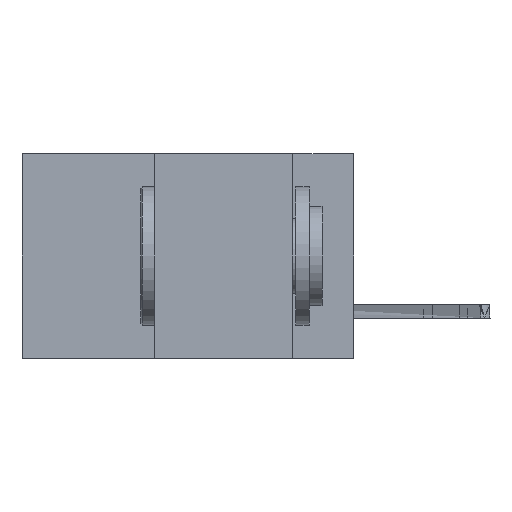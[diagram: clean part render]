
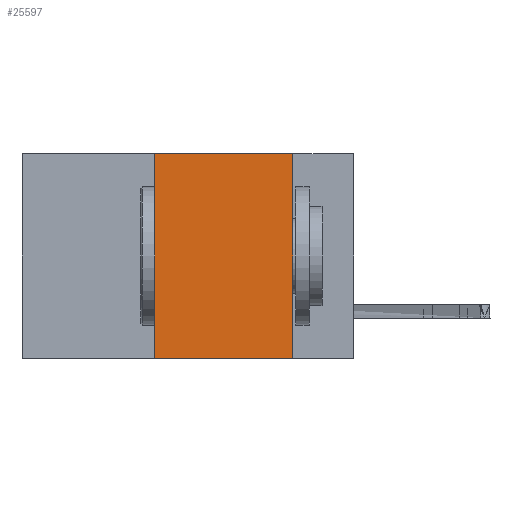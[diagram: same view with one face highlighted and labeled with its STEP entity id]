
A CAD part, left-side view. The second image highlights one B-rep face of the part: STEP entity #25597.
In plain terms, the highlighted planar face has unit normal (-1, 0, 0).
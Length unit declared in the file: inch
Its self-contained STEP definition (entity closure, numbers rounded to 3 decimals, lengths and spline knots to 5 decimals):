
#1779 = CARTESIAN_POINT ( 'NONE',  ( 0., 0.36, 0. ) ) ;
#3085 = CARTESIAN_POINT ( 'NONE',  ( 0., 0.36, -0.37 ) ) ;
#4641 = ORIENTED_EDGE ( 'NONE', *, *, #24903, .F. ) ;
#5412 = VERTEX_POINT ( 'NONE', #3085 ) ;
#5747 = LINE ( 'NONE', #26529, #12934 ) ;
#5913 = CARTESIAN_POINT ( 'NONE',  ( 0., 0.11, -0.37 ) ) ;
#6704 = LINE ( 'NONE', #31132, #27603 ) ;
#7426 = DIRECTION ( 'NONE',  ( 0., -1., 0. ) ) ;
#8399 = VERTEX_POINT ( 'NONE', #32566 ) ;
#8525 = CARTESIAN_POINT ( 'NONE',  ( 0., 0.6, -0.37 ) ) ;
#8877 = VERTEX_POINT ( 'NONE', #1779 ) ;
#10128 = CARTESIAN_POINT ( 'NONE',  ( 0., 0.36, 0. ) ) ;
#11796 = EDGE_LOOP ( 'NONE', ( #4641, #28111, #28960, #24326 ) ) ;
#12002 = DIRECTION ( 'NONE',  ( 0., 0., -1. ) ) ;
#12072 = PLANE ( 'NONE',  #30386 ) ;
#12934 = VECTOR ( 'NONE', #7426, 39.37008 ) ;
#15010 = VECTOR ( 'NONE', #29236, 39.37008 ) ;
#15148 = EDGE_CURVE ( 'NONE', #8877, #8399, #5747, .T. ) ;
#17596 = DIRECTION ( 'NONE',  ( 0., 0., -1. ) ) ;
#21464 = LINE ( 'NONE', #10128, #15010 ) ;
#22756 = VERTEX_POINT ( 'NONE', #5913 ) ;
#24326 = ORIENTED_EDGE ( 'NONE', *, *, #26042, .T. ) ;
#24570 = VECTOR ( 'NONE', #24899, 39.37008 ) ;
#24899 = DIRECTION ( 'NONE',  ( 0., -1., 0. ) ) ;
#24903 = EDGE_CURVE ( 'NONE', #8399, #22756, #6704, .T. ) ;
#25463 = FACE_OUTER_BOUND ( 'NONE', #11796, .T. ) ;
#25597 = ADVANCED_FACE ( 'NONE', ( #25463 ), #12072, .F. ) ;
#26042 = EDGE_CURVE ( 'NONE', #5412, #22756, #31771, .T. ) ;
#26529 = CARTESIAN_POINT ( 'NONE',  ( 0., 0.6, 0. ) ) ;
#27603 = VECTOR ( 'NONE', #12002, 39.37008 ) ;
#28111 = ORIENTED_EDGE ( 'NONE', *, *, #15148, .F. ) ;
#28960 = ORIENTED_EDGE ( 'NONE', *, *, #34019, .F. ) ;
#29236 = DIRECTION ( 'NONE',  ( 0., 0., 1. ) ) ;
#30386 = AXIS2_PLACEMENT_3D ( 'NONE', #31200, #33966, #17596 ) ;
#31132 = CARTESIAN_POINT ( 'NONE',  ( 0., 0.11, 0. ) ) ;
#31200 = CARTESIAN_POINT ( 'NONE',  ( 0., 0.6, 0. ) ) ;
#31771 = LINE ( 'NONE', #8525, #24570 ) ;
#32566 = CARTESIAN_POINT ( 'NONE',  ( 0., 0.11, 0. ) ) ;
#33966 = DIRECTION ( 'NONE',  ( 1., 0., 0. ) ) ;
#34019 = EDGE_CURVE ( 'NONE', #5412, #8877, #21464, .T. ) ;
